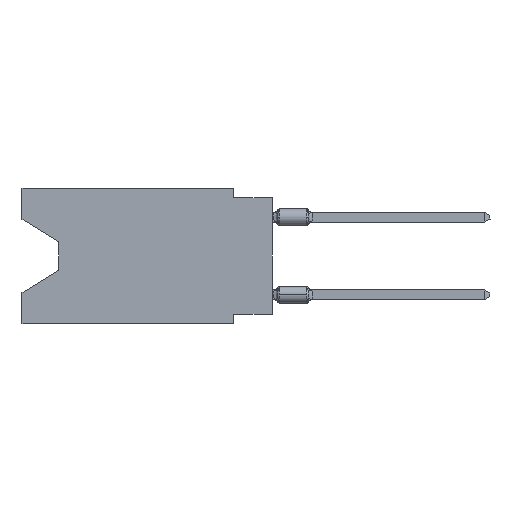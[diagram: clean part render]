
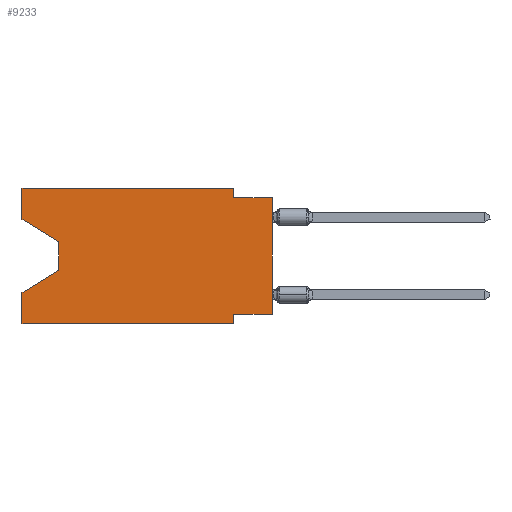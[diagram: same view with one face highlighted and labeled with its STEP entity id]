
A CAD part, left-side view. The second image highlights one B-rep face of the part: STEP entity #9233.
In plain terms, the highlighted planar face has unit normal (-1, 0, 0).
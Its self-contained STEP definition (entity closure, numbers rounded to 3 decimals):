
#7 = EDGE_CURVE ( 'NONE', #5698, #12604, #18111, .T. ) ;
#844 = VECTOR ( 'NONE', #34683, 1000. ) ;
#1426 = CARTESIAN_POINT ( 'NONE',  ( 0., 2.54, 0. ) ) ;
#1574 = CARTESIAN_POINT ( 'NONE',  ( 0., 13.97, -3.505 ) ) ;
#1587 = LINE ( 'NONE', #7474, #34932 ) ;
#1644 = CARTESIAN_POINT ( 'NONE',  ( 0., 16.383, -8.89 ) ) ;
#2502 = ORIENTED_EDGE ( 'NONE', *, *, #15885, .T. ) ;
#3833 = DIRECTION ( 'NONE',  ( 0., 0., -1. ) ) ;
#4148 = EDGE_CURVE ( 'NONE', #15141, #12604, #32024, .T. ) ;
#4537 = ORIENTED_EDGE ( 'NONE', *, *, #19460, .F. ) ;
#5094 = DIRECTION ( 'NONE',  ( 0., -1., 0. ) ) ;
#5477 = CARTESIAN_POINT ( 'NONE',  ( 0., 13.97, -5.385 ) ) ;
#5698 = VERTEX_POINT ( 'NONE', #19721 ) ;
#6061 = EDGE_CURVE ( 'NONE', #30729, #20213, #38594, .T. ) ;
#6180 = ORIENTED_EDGE ( 'NONE', *, *, #37045, .F. ) ;
#6303 = CARTESIAN_POINT ( 'NONE',  ( 0., 16.383, 0. ) ) ;
#6525 = LINE ( 'NONE', #32352, #11689 ) ;
#6714 = VECTOR ( 'NONE', #38262, 1000. ) ;
#7474 = CARTESIAN_POINT ( 'NONE',  ( 0., 16.383, -2.038 ) ) ;
#8225 = CARTESIAN_POINT ( 'NONE',  ( 0., 2.54, 0. ) ) ;
#8421 = AXIS2_PLACEMENT_3D ( 'NONE', #27445, #40487, #3833 ) ;
#8493 = DIRECTION ( 'NONE',  ( 0., -1., 0. ) ) ;
#8893 = VERTEX_POINT ( 'NONE', #15534 ) ;
#9233 = ADVANCED_FACE ( 'NONE', ( #14228 ), #37240, .F. ) ;
#10069 = CARTESIAN_POINT ( 'NONE',  ( 0., 2.54, -8.89 ) ) ;
#10307 = CARTESIAN_POINT ( 'NONE',  ( 0., 13.97, -3.505 ) ) ;
#10435 = ORIENTED_EDGE ( 'NONE', *, *, #13746, .T. ) ;
#10623 = VERTEX_POINT ( 'NONE', #27699 ) ;
#10712 = LINE ( 'NONE', #37197, #41919 ) ;
#11689 = VECTOR ( 'NONE', #29507, 1000. ) ;
#12401 = LINE ( 'NONE', #1574, #34321 ) ;
#12499 = DIRECTION ( 'NONE',  ( 0., 0., -1. ) ) ;
#12604 = VERTEX_POINT ( 'NONE', #10069 ) ;
#13028 = DIRECTION ( 'NONE',  ( 0., -1., 0. ) ) ;
#13066 = ORIENTED_EDGE ( 'NONE', *, *, #13630, .F. ) ;
#13630 = EDGE_CURVE ( 'NONE', #20213, #28789, #35186, .T. ) ;
#13746 = EDGE_CURVE ( 'NONE', #22341, #16025, #12401, .T. ) ;
#14228 = FACE_OUTER_BOUND ( 'NONE', #33149, .T. ) ;
#14422 = ORIENTED_EDGE ( 'NONE', *, *, #6061, .F. ) ;
#15054 = CARTESIAN_POINT ( 'NONE',  ( 0., 16.383, 0. ) ) ;
#15141 = VERTEX_POINT ( 'NONE', #34288 ) ;
#15258 = LINE ( 'NONE', #15054, #6714 ) ;
#15338 = VERTEX_POINT ( 'NONE', #38624 ) ;
#15534 = CARTESIAN_POINT ( 'NONE',  ( 0., 16.383, -2.038 ) ) ;
#15885 = EDGE_CURVE ( 'NONE', #8893, #22341, #1587, .T. ) ;
#16025 = VERTEX_POINT ( 'NONE', #5477 ) ;
#16261 = CARTESIAN_POINT ( 'NONE',  ( 0., 0., -0.635 ) ) ;
#16795 = ORIENTED_EDGE ( 'NONE', *, *, #7, .T. ) ;
#17156 = VECTOR ( 'NONE', #13028, 1000. ) ;
#17230 = DIRECTION ( 'NONE',  ( 0., 0., 1. ) ) ;
#17913 = ORIENTED_EDGE ( 'NONE', *, *, #36346, .F. ) ;
#18111 = LINE ( 'NONE', #1644, #38014 ) ;
#18358 = LINE ( 'NONE', #31594, #38457 ) ;
#19460 = EDGE_CURVE ( 'NONE', #5698, #15338, #10712, .T. ) ;
#19721 = CARTESIAN_POINT ( 'NONE',  ( 0., 16.383, -8.89 ) ) ;
#20213 = VERTEX_POINT ( 'NONE', #29902 ) ;
#20403 = VECTOR ( 'NONE', #12499, 1000. ) ;
#22341 = VERTEX_POINT ( 'NONE', #10307 ) ;
#23205 = LINE ( 'NONE', #6303, #17156 ) ;
#23930 = DIRECTION ( 'NONE',  ( 0., -0.855, -0.519 ) ) ;
#25168 = CARTESIAN_POINT ( 'NONE',  ( 0., 0., -0.635 ) ) ;
#25656 = CARTESIAN_POINT ( 'NONE',  ( 0., 13.97, -5.385 ) ) ;
#25708 = CARTESIAN_POINT ( 'NONE',  ( 0., 2.54, -8.89 ) ) ;
#26636 = VECTOR ( 'NONE', #38503, 1000. ) ;
#27445 = CARTESIAN_POINT ( 'NONE',  ( 0., 16.383, 0. ) ) ;
#27699 = CARTESIAN_POINT ( 'NONE',  ( 0., 0., -8.255 ) ) ;
#27804 = ORIENTED_EDGE ( 'NONE', *, *, #4148, .F. ) ;
#28763 = DIRECTION ( 'NONE',  ( 0., 1., 0. ) ) ;
#28789 = VERTEX_POINT ( 'NONE', #16261 ) ;
#29507 = DIRECTION ( 'NONE',  ( 0., 0., 1. ) ) ;
#29902 = CARTESIAN_POINT ( 'NONE',  ( 0., 2.54, -0.635 ) ) ;
#30486 = EDGE_CURVE ( 'NONE', #10623, #15141, #18358, .T. ) ;
#30505 = ORIENTED_EDGE ( 'NONE', *, *, #38622, .T. ) ;
#30729 = VERTEX_POINT ( 'NONE', #1426 ) ;
#31594 = CARTESIAN_POINT ( 'NONE',  ( 0., 0., -8.255 ) ) ;
#32024 = LINE ( 'NONE', #25708, #20403 ) ;
#32127 = DIRECTION ( 'NONE',  ( 0., 0., -1. ) ) ;
#32302 = ORIENTED_EDGE ( 'NONE', *, *, #30486, .F. ) ;
#32352 = CARTESIAN_POINT ( 'NONE',  ( 0., 0., 0. ) ) ;
#33149 = EDGE_LOOP ( 'NONE', ( #2502, #10435, #41785, #4537, #16795, #27804, #32302, #30505, #13066, #14422, #6180, #17913 ) ) ;
#34288 = CARTESIAN_POINT ( 'NONE',  ( 0., 2.54, -8.255 ) ) ;
#34321 = VECTOR ( 'NONE', #32127, 1000. ) ;
#34683 = DIRECTION ( 'NONE',  ( 0., 0., -1. ) ) ;
#34932 = VECTOR ( 'NONE', #23930, 1000. ) ;
#35186 = LINE ( 'NONE', #25168, #42660 ) ;
#36346 = EDGE_CURVE ( 'NONE', #8893, #38485, #15258, .T. ) ;
#37045 = EDGE_CURVE ( 'NONE', #38485, #30729, #23205, .T. ) ;
#37197 = CARTESIAN_POINT ( 'NONE',  ( 0., 16.383, 0. ) ) ;
#37240 = PLANE ( 'NONE',  #8421 ) ;
#38014 = VECTOR ( 'NONE', #5094, 1000. ) ;
#38017 = CARTESIAN_POINT ( 'NONE',  ( 0., 16.383, 0. ) ) ;
#38262 = DIRECTION ( 'NONE',  ( 0., 0., 1. ) ) ;
#38457 = VECTOR ( 'NONE', #28763, 1000. ) ;
#38485 = VERTEX_POINT ( 'NONE', #38017 ) ;
#38503 = DIRECTION ( 'NONE',  ( 0., 0.855, -0.519 ) ) ;
#38594 = LINE ( 'NONE', #8225, #844 ) ;
#38622 = EDGE_CURVE ( 'NONE', #10623, #28789, #6525, .T. ) ;
#38624 = CARTESIAN_POINT ( 'NONE',  ( 0., 16.383, -6.852 ) ) ;
#39149 = LINE ( 'NONE', #25656, #26636 ) ;
#39810 = EDGE_CURVE ( 'NONE', #16025, #15338, #39149, .T. ) ;
#40487 = DIRECTION ( 'NONE',  ( 1., 0., 0. ) ) ;
#41785 = ORIENTED_EDGE ( 'NONE', *, *, #39810, .T. ) ;
#41919 = VECTOR ( 'NONE', #17230, 1000. ) ;
#42660 = VECTOR ( 'NONE', #8493, 1000. ) ;
